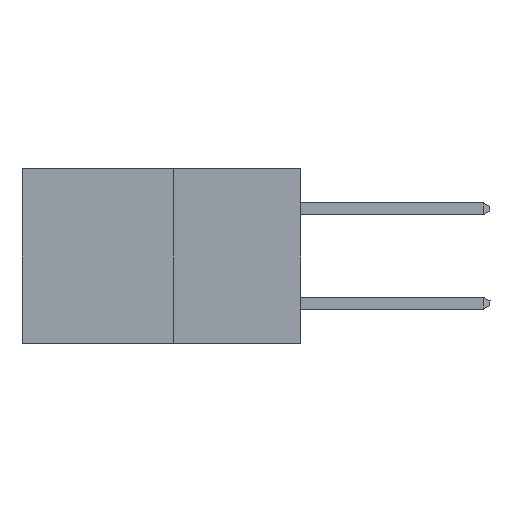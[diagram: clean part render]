
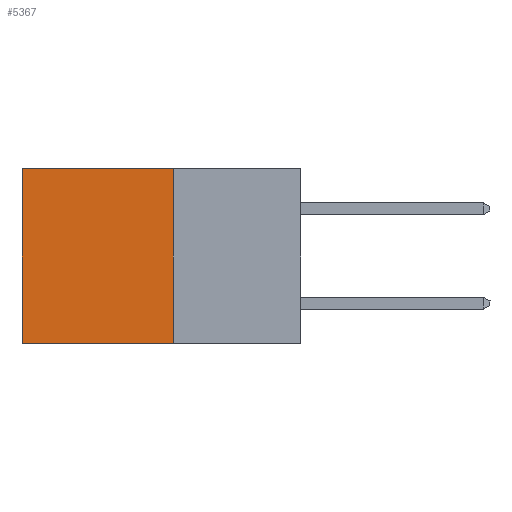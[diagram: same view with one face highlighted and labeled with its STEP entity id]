
A CAD part, left-side view. The second image highlights one B-rep face of the part: STEP entity #5367.
In plain terms, the highlighted planar face has unit normal (-1, 0, 0).
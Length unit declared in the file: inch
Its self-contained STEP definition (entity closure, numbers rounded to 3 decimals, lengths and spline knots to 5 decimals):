
#561 = VECTOR ( 'NONE', #20038, 39.37008 ) ;
#578 = ORIENTED_EDGE ( 'NONE', *, *, #4213, .F. ) ;
#765 = VERTEX_POINT ( 'NONE', #28018 ) ;
#3948 = VECTOR ( 'NONE', #23226, 39.37008 ) ;
#4213 = EDGE_CURVE ( 'NONE', #765, #9586, #14671, .T. ) ;
#5367 = ADVANCED_FACE ( 'NONE', ( #27124 ), #7421, .F. ) ;
#7314 = DIRECTION ( 'NONE',  ( 0., 0., -1. ) ) ;
#7323 = VERTEX_POINT ( 'NONE', #20200 ) ;
#7346 = DIRECTION ( 'NONE',  ( 1., 0., 0. ) ) ;
#7388 = CARTESIAN_POINT ( 'NONE',  ( 0.277, 0.27, -0.37 ) ) ;
#7421 = PLANE ( 'NONE',  #26354 ) ;
#7513 = LINE ( 'NONE', #14823, #561 ) ;
#7529 = CARTESIAN_POINT ( 'NONE',  ( 0.277, 0.59, -0.37 ) ) ;
#7742 = VECTOR ( 'NONE', #29788, 39.37008 ) ;
#9586 = VERTEX_POINT ( 'NONE', #23600 ) ;
#10888 = DIRECTION ( 'NONE',  ( 0., 1., 0. ) ) ;
#10959 = LINE ( 'NONE', #7529, #3948 ) ;
#11964 = ORIENTED_EDGE ( 'NONE', *, *, #23417, .T. ) ;
#12058 = EDGE_CURVE ( 'NONE', #22882, #7323, #10959, .T. ) ;
#13679 = LINE ( 'NONE', #31483, #26579 ) ;
#14671 = LINE ( 'NONE', #29916, #7742 ) ;
#14823 = CARTESIAN_POINT ( 'NONE',  ( 0.277, 0.27, 0. ) ) ;
#16659 = EDGE_LOOP ( 'NONE', ( #21156, #30426, #578, #11964 ) ) ;
#20038 = DIRECTION ( 'NONE',  ( 0., 1., 0. ) ) ;
#20200 = CARTESIAN_POINT ( 'NONE',  ( 0.277, 0.59, -0.37 ) ) ;
#21156 = ORIENTED_EDGE ( 'NONE', *, *, #12058, .T. ) ;
#22882 = VERTEX_POINT ( 'NONE', #23355 ) ;
#23226 = DIRECTION ( 'NONE',  ( 0., 0., -1. ) ) ;
#23355 = CARTESIAN_POINT ( 'NONE',  ( 0.277, 0.59, 0. ) ) ;
#23417 = EDGE_CURVE ( 'NONE', #765, #22882, #7513, .T. ) ;
#23600 = CARTESIAN_POINT ( 'NONE',  ( 0.277, 0.27, -0.37 ) ) ;
#26354 = AXIS2_PLACEMENT_3D ( 'NONE', #7388, #7346, #7314 ) ;
#26579 = VECTOR ( 'NONE', #10888, 39.37008 ) ;
#27124 = FACE_OUTER_BOUND ( 'NONE', #16659, .T. ) ;
#28018 = CARTESIAN_POINT ( 'NONE',  ( 0.277, 0.27, 0. ) ) ;
#29788 = DIRECTION ( 'NONE',  ( 0., 0., -1. ) ) ;
#29916 = CARTESIAN_POINT ( 'NONE',  ( 0.277, 0.27, -0.37 ) ) ;
#30426 = ORIENTED_EDGE ( 'NONE', *, *, #32864, .F. ) ;
#31483 = CARTESIAN_POINT ( 'NONE',  ( 0.277, 0.27, -0.37 ) ) ;
#32864 = EDGE_CURVE ( 'NONE', #9586, #7323, #13679, .T. ) ;
